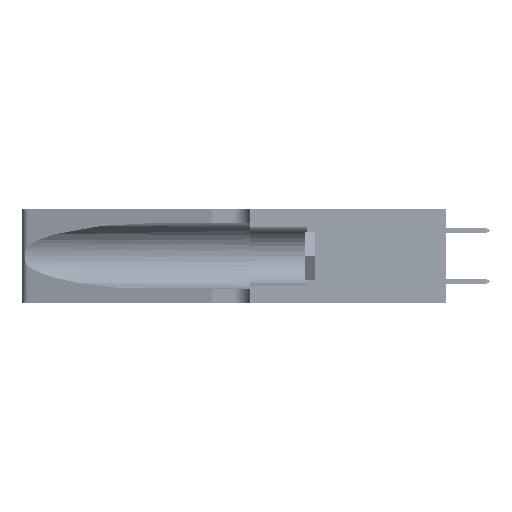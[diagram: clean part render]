
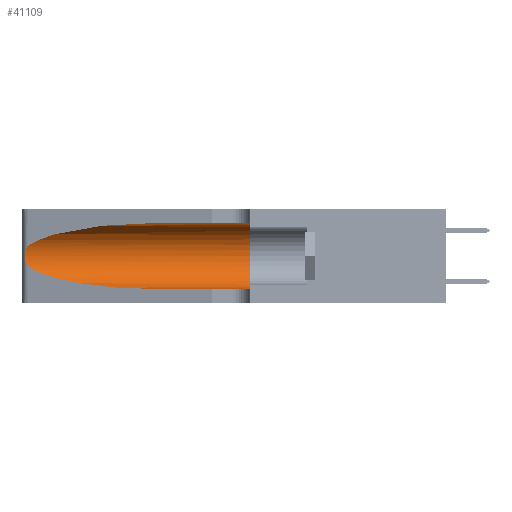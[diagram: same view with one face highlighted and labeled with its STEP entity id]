
A CAD part, left-side view. The second image highlights one B-rep face of the part: STEP entity #41109.
In plain terms, the highlighted cylindrical face has radius 3.308 mm (diameter 6.617 mm), a partial arc.
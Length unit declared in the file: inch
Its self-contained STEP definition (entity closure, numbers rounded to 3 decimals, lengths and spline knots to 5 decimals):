
#630 = CARTESIAN_POINT ( 'NONE',  ( 0.25487, 1.22718, 0.14631 ) ) ;
#1389 = VERTEX_POINT ( 'NONE', #27588 ) ;
#1497 = CARTESIAN_POINT ( 'NONE',  ( 0.1305, 1.61858, 0.05475 ) ) ;
#1521 = EDGE_CURVE ( 'NONE', #37454, #5999, #34131, .T. ) ;
#1554 = CARTESIAN_POINT ( 'NONE',  ( 0.1305, 0.35, 0.185 ) ) ;
#4301 = VECTOR ( 'NONE', #8443, 39.37008 ) ;
#4424 = CARTESIAN_POINT ( 'NONE',  ( 0.25639, 1.23186, 0.15144 ) ) ;
#5496 = CARTESIAN_POINT ( 'NONE',  ( 0.1305, 0.72297, 0.05475 ) ) ;
#5999 = VERTEX_POINT ( 'NONE', #7889 ) ;
#7290 = EDGE_CURVE ( 'NONE', #42714, #1389, #25236, .T. ) ;
#7889 = CARTESIAN_POINT ( 'NONE',  ( 0.1305, 0.35, 0.05475 ) ) ;
#8323 = CARTESIAN_POINT ( 'NONE',  ( 0.25639, 1.23184, 0.21858 ) ) ;
#8443 = DIRECTION ( 'NONE',  ( 0., -1., 0. ) ) ;
#11295 = CARTESIAN_POINT ( 'NONE',  ( 0.25854, 1.2359, 0.20912 ) ) ;
#11379 = ORIENTED_EDGE ( 'NONE', *, *, #41909, .F. ) ;
#11720 = CIRCLE ( 'NONE', #29158, 0.13025 ) ;
#11782 = CARTESIAN_POINT ( 'NONE',  ( 0.25555, 1.22994, 0.2215 ) ) ;
#12425 = CARTESIAN_POINT ( 'NONE',  ( 0.25487, 1.22718, 0.22369 ) ) ;
#12834 =( BOUNDED_CURVE ( )  B_SPLINE_CURVE ( 3, ( #22812, #33912, #15728, #12425 ),
 .UNSPECIFIED., .F., .T. ) 
 B_SPLINE_CURVE_WITH_KNOTS ( ( 4, 4 ),
 ( 1.5708, 2.84003 ),
 .UNSPECIFIED. ) 
 CURVE ( )  GEOMETRIC_REPRESENTATION_ITEM ( )  RATIONAL_B_SPLINE_CURVE ( ( 1., 0.87, 0.87, 1. ) ) 
 REPRESENTATION_ITEM ( '' )  );
#13082 = VERTEX_POINT ( 'NONE', #38312 ) ;
#14253 = ORIENTED_EDGE ( 'NONE', *, *, #30816, .T. ) ;
#14916 = CARTESIAN_POINT ( 'NONE',  ( 0.25555, 1.22993, 0.14849 ) ) ;
#15078 = CARTESIAN_POINT ( 'NONE',  ( 0.25856, 1.23593, 0.16098 ) ) ;
#15728 = CARTESIAN_POINT ( 'NONE',  ( 0.2373, 1.15595, 0.28018 ) ) ;
#17684 = CARTESIAN_POINT ( 'NONE',  ( 0.1305, 0.35, 0.31525 ) ) ;
#18350 = LINE ( 'NONE', #26980, #4301 ) ;
#19011 = CARTESIAN_POINT ( 'NONE',  ( 0.25787, 1.23484, 0.2124 ) ) ;
#19620 = DIRECTION ( 'NONE',  ( 0., 1., 0. ) ) ;
#20841 = ORIENTED_EDGE ( 'NONE', *, *, #1521, .T. ) ;
#21128 = EDGE_LOOP ( 'NONE', ( #14253, #37899, #30135, #20841, #22679, #11379 ) ) ;
#22014 = CARTESIAN_POINT ( 'NONE',  ( 0.25487, 1.22718, 0.22369 ) ) ;
#22679 = ORIENTED_EDGE ( 'NONE', *, *, #40577, .F. ) ;
#22812 = CARTESIAN_POINT ( 'NONE',  ( 0.1305, 0.72297, 0.31525 ) ) ;
#24352 = AXIS2_PLACEMENT_3D ( 'NONE', #26024, #26179, #29287 ) ;
#24527 = CARTESIAN_POINT ( 'NONE',  ( 0.1305, 0.72297, 0.05475 ) ) ;
#25236 = B_SPLINE_CURVE_WITH_KNOTS ( 'NONE', 3,
 ( #22014, #11782, #8323, #19011, #11295, #36874, #36401, #32977, #44105, #15078, #36718, #4424, #14916, #630 ),
 .UNSPECIFIED., .F., .F.,
 ( 4, 2, 2, 2, 2, 2, 4 ),
 ( 0., 0.00027, 0.00053, 0.00107, 0.0016, 0.00187, 0.00214 ),
 .UNSPECIFIED. ) ;
#26024 = CARTESIAN_POINT ( 'NONE',  ( 0.1305, 1.61858, 0.185 ) ) ;
#26179 = DIRECTION ( 'NONE',  ( 0., -1., 0. ) ) ;
#26980 = CARTESIAN_POINT ( 'NONE',  ( 0.1305, 1.61858, 0.31525 ) ) ;
#26991 = CARTESIAN_POINT ( 'NONE',  ( 0.2373, 1.15595, 0.08982 ) ) ;
#27588 = CARTESIAN_POINT ( 'NONE',  ( 0.25487, 1.22718, 0.14631 ) ) ;
#29158 = AXIS2_PLACEMENT_3D ( 'NONE', #1554, #19620, #30436 ) ;
#29287 = DIRECTION ( 'NONE',  ( 0., 0., -1. ) ) ;
#30135 = ORIENTED_EDGE ( 'NONE', *, *, #40749, .T. ) ;
#30436 = DIRECTION ( 'NONE',  ( 0., 0., 1. ) ) ;
#30816 = EDGE_CURVE ( 'NONE', #13082, #42714, #12834, .T. ) ;
#31203 = CARTESIAN_POINT ( 'NONE',  ( 0.18966, 0.96281, 0.05475 ) ) ;
#32977 = CARTESIAN_POINT ( 'NONE',  ( 0.26075, 1.23896, 0.178 ) ) ;
#33912 = CARTESIAN_POINT ( 'NONE',  ( 0.18966, 0.96281, 0.31525 ) ) ;
#34131 = LINE ( 'NONE', #1497, #34707 ) ;
#34707 = VECTOR ( 'NONE', #35543, 39.37008 ) ;
#35543 = DIRECTION ( 'NONE',  ( 0., -1., 0. ) ) ;
#36401 = CARTESIAN_POINT ( 'NONE',  ( 0.26075, 1.23896, 0.19203 ) ) ;
#36718 = CARTESIAN_POINT ( 'NONE',  ( 0.25789, 1.23486, 0.15765 ) ) ;
#36874 = CARTESIAN_POINT ( 'NONE',  ( 0.26018, 1.23835, 0.19895 ) ) ;
#37454 = VERTEX_POINT ( 'NONE', #24527 ) ;
#37899 = ORIENTED_EDGE ( 'NONE', *, *, #7290, .T. ) ;
#38312 = CARTESIAN_POINT ( 'NONE',  ( 0.1305, 0.72297, 0.31525 ) ) ;
#38465 = CARTESIAN_POINT ( 'NONE',  ( 0.25487, 1.22718, 0.22369 ) ) ;
#39274 =( BOUNDED_CURVE ( )  B_SPLINE_CURVE ( 3, ( #41862, #26991, #31203, #5496 ),
 .UNSPECIFIED., .F., .T. ) 
 B_SPLINE_CURVE_WITH_KNOTS ( ( 4, 4 ),
 ( 3.44316, 4.71239 ),
 .UNSPECIFIED. ) 
 CURVE ( )  GEOMETRIC_REPRESENTATION_ITEM ( )  RATIONAL_B_SPLINE_CURVE ( ( 1., 0.87, 0.87, 1. ) ) 
 REPRESENTATION_ITEM ( '' )  );
#40577 = EDGE_CURVE ( 'NONE', #41003, #5999, #11720, .T. ) ;
#40749 = EDGE_CURVE ( 'NONE', #1389, #37454, #39274, .T. ) ;
#41003 = VERTEX_POINT ( 'NONE', #17684 ) ;
#41109 = ADVANCED_FACE ( 'NONE', ( #45328 ), #44233, .F. ) ;
#41862 = CARTESIAN_POINT ( 'NONE',  ( 0.25487, 1.22718, 0.14631 ) ) ;
#41909 = EDGE_CURVE ( 'NONE', #13082, #41003, #18350, .T. ) ;
#42714 = VERTEX_POINT ( 'NONE', #38465 ) ;
#44105 = CARTESIAN_POINT ( 'NONE',  ( 0.26017, 1.23833, 0.17102 ) ) ;
#44233 = CYLINDRICAL_SURFACE ( 'NONE', #24352, 0.13025 ) ;
#45328 = FACE_OUTER_BOUND ( 'NONE', #21128, .T. ) ;
